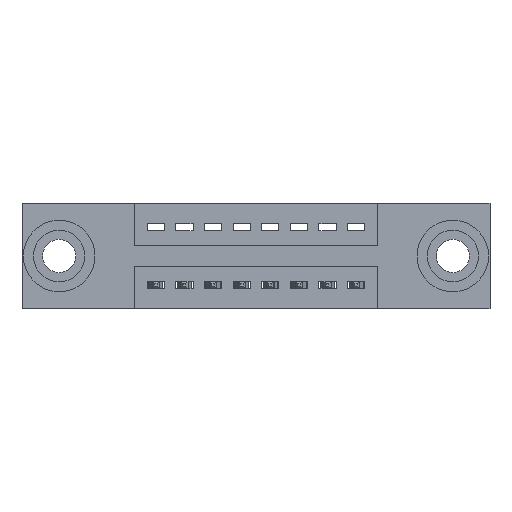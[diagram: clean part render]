
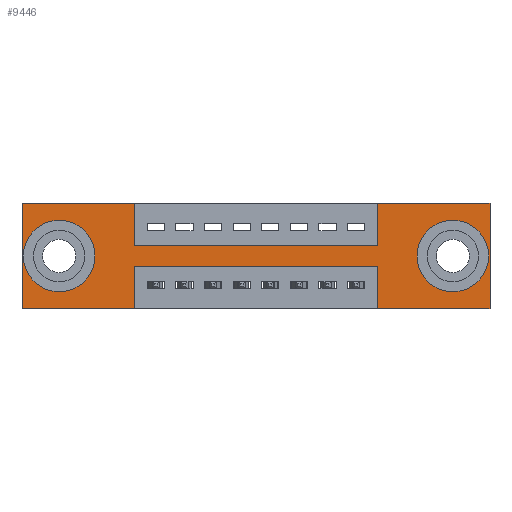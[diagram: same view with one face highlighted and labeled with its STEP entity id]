
A CAD part, front view. The second image highlights one B-rep face of the part: STEP entity #9446.
In plain terms, the highlighted planar face has unit normal (0, -1, 0).
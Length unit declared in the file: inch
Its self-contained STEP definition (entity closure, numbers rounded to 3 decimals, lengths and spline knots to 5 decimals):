
#60 = VERTEX_POINT ( 'NONE', #6578 ) ;
#128 = DIRECTION ( 'NONE',  ( 0., 0., -1. ) ) ;
#153 = VERTEX_POINT ( 'NONE', #2269 ) ;
#289 = CARTESIAN_POINT ( 'NONE',  ( 0.3925, 0., -0.37 ) ) ;
#307 = VERTEX_POINT ( 'NONE', #1659 ) ;
#315 = CARTESIAN_POINT ( 'NONE',  ( 0.3925, 0., -0.15 ) ) ;
#331 = DIRECTION ( 'NONE',  ( 0., 0., 1. ) ) ;
#433 = EDGE_LOOP ( 'NONE', ( #3900, #6845 ) ) ;
#526 = LINE ( 'NONE', #1636, #4480 ) ;
#568 = CARTESIAN_POINT ( 'NONE',  ( 0., 0., 0. ) ) ;
#643 = CARTESIAN_POINT ( 'NONE',  ( 0.3925, 0., 0. ) ) ;
#735 = ORIENTED_EDGE ( 'NONE', *, *, #931, .T. ) ;
#931 = EDGE_CURVE ( 'NONE', #4063, #60, #10471, .T. ) ;
#942 = ORIENTED_EDGE ( 'NONE', *, *, #6982, .F. ) ;
#1045 = ORIENTED_EDGE ( 'NONE', *, *, #2650, .F. ) ;
#1110 = DIRECTION ( 'NONE',  ( 0., 0., -1. ) ) ;
#1245 = CARTESIAN_POINT ( 'NONE',  ( 1.635, 0., -0.37 ) ) ;
#1304 = VERTEX_POINT ( 'NONE', #8919 ) ;
#1343 = CARTESIAN_POINT ( 'NONE',  ( 1.2425, 0., 0. ) ) ;
#1618 = CARTESIAN_POINT ( 'NONE',  ( 0.3925, 0., -0.22 ) ) ;
#1636 = CARTESIAN_POINT ( 'NONE',  ( 0., 0., 0. ) ) ;
#1659 = CARTESIAN_POINT ( 'NONE',  ( 1.2425, 0., -0.37 ) ) ;
#1731 = DIRECTION ( 'NONE',  ( -1., 0., 0. ) ) ;
#1753 = VECTOR ( 'NONE', #4052, 39.37008 ) ;
#1759 = ORIENTED_EDGE ( 'NONE', *, *, #3820, .F. ) ;
#1963 = DIRECTION ( 'NONE',  ( 1., 0., 0. ) ) ;
#1981 = CARTESIAN_POINT ( 'NONE',  ( 1.505, 0., -0.185 ) ) ;
#2000 = CARTESIAN_POINT ( 'NONE',  ( 0.13, 0., -0.107 ) ) ;
#2029 = DIRECTION ( 'NONE',  ( -1., 0., 0. ) ) ;
#2114 = LINE ( 'NONE', #1618, #9882 ) ;
#2201 = ORIENTED_EDGE ( 'NONE', *, *, #4584, .F. ) ;
#2204 = DIRECTION ( 'NONE',  ( 0., 0., 1. ) ) ;
#2269 = CARTESIAN_POINT ( 'NONE',  ( 1.2425, 0., -0.15 ) ) ;
#2284 = FACE_BOUND ( 'NONE', #433, .T. ) ;
#2317 = LINE ( 'NONE', #9646, #4358 ) ;
#2338 = DIRECTION ( 'NONE',  ( 0., 0., -1. ) ) ;
#2351 = VECTOR ( 'NONE', #2029, 39.37008 ) ;
#2459 = DIRECTION ( 'NONE',  ( 1., 0., 0. ) ) ;
#2521 = EDGE_LOOP ( 'NONE', ( #5849, #1045, #10937, #2791, #942, #10376, #9166, #8286, #11074, #4075, #2201, #1759 ) ) ;
#2650 = EDGE_CURVE ( 'NONE', #6185, #4301, #2114, .T. ) ;
#2688 = DIRECTION ( 'NONE',  ( 0., 0., 1. ) ) ;
#2727 = CARTESIAN_POINT ( 'NONE',  ( 0.13, 0., -0.185 ) ) ;
#2745 = LINE ( 'NONE', #315, #7666 ) ;
#2784 = CARTESIAN_POINT ( 'NONE',  ( 1.2425, 0., -0.37 ) ) ;
#2791 = ORIENTED_EDGE ( 'NONE', *, *, #5327, .F. ) ;
#3038 = VERTEX_POINT ( 'NONE', #1245 ) ;
#3396 = VECTOR ( 'NONE', #2204, 39.37008 ) ;
#3820 = EDGE_CURVE ( 'NONE', #10307, #1304, #5655, .T. ) ;
#3857 = EDGE_CURVE ( 'NONE', #6645, #8195, #11081, .T. ) ;
#3900 = ORIENTED_EDGE ( 'NONE', *, *, #8445, .T. ) ;
#3925 = LINE ( 'NONE', #2784, #8863 ) ;
#4052 = DIRECTION ( 'NONE',  ( -1., 0., 0. ) ) ;
#4058 = CARTESIAN_POINT ( 'NONE',  ( 1.505, 0., -0.107 ) ) ;
#4063 = VERTEX_POINT ( 'NONE', #2000 ) ;
#4065 = LINE ( 'NONE', #8425, #1753 ) ;
#4075 = ORIENTED_EDGE ( 'NONE', *, *, #8990, .F. ) ;
#4301 = VERTEX_POINT ( 'NONE', #6123 ) ;
#4358 = VECTOR ( 'NONE', #11283, 39.37008 ) ;
#4439 = CARTESIAN_POINT ( 'NONE',  ( 0.3925, 0., -0.37 ) ) ;
#4464 = AXIS2_PLACEMENT_3D ( 'NONE', #5809, #7580, #2338 ) ;
#4480 = VECTOR ( 'NONE', #2459, 39.37008 ) ;
#4584 = EDGE_CURVE ( 'NONE', #1304, #7609, #8911, .T. ) ;
#4637 = EDGE_LOOP ( 'NONE', ( #735, #5672 ) ) ;
#4876 = AXIS2_PLACEMENT_3D ( 'NONE', #10979, #5778, #6798 ) ;
#4888 = PLANE ( 'NONE',  #4876 ) ;
#5173 = AXIS2_PLACEMENT_3D ( 'NONE', #1981, #10635, #128 ) ;
#5235 = VERTEX_POINT ( 'NONE', #643 ) ;
#5327 = EDGE_CURVE ( 'NONE', #3038, #307, #4065, .T. ) ;
#5449 = DIRECTION ( 'NONE',  ( 0., 0., 1. ) ) ;
#5454 = DIRECTION ( 'NONE',  ( 1., 0., 0. ) ) ;
#5500 = LINE ( 'NONE', #8030, #8903 ) ;
#5539 = DIRECTION ( 'NONE',  ( 0., 1., 0. ) ) ;
#5655 = LINE ( 'NONE', #7265, #2351 ) ;
#5672 = ORIENTED_EDGE ( 'NONE', *, *, #10271, .T. ) ;
#5778 = DIRECTION ( 'NONE',  ( 0., -1., 0. ) ) ;
#5809 = CARTESIAN_POINT ( 'NONE',  ( 1.505, 0., -0.185 ) ) ;
#5849 = ORIENTED_EDGE ( 'NONE', *, *, #6382, .F. ) ;
#5914 = LINE ( 'NONE', #4439, #7551 ) ;
#5947 = VERTEX_POINT ( 'NONE', #9475 ) ;
#6069 = CARTESIAN_POINT ( 'NONE',  ( 0., 0., 0. ) ) ;
#6123 = CARTESIAN_POINT ( 'NONE',  ( 0.3925, 0., -0.22 ) ) ;
#6124 = FACE_BOUND ( 'NONE', #4637, .T. ) ;
#6185 = VERTEX_POINT ( 'NONE', #9201 ) ;
#6382 = EDGE_CURVE ( 'NONE', #4301, #10307, #5914, .T. ) ;
#6578 = CARTESIAN_POINT ( 'NONE',  ( 0.13, 0., -0.263 ) ) ;
#6592 = DIRECTION ( 'NONE',  ( 0., 0., 1. ) ) ;
#6645 = VERTEX_POINT ( 'NONE', #10576 ) ;
#6713 = AXIS2_PLACEMENT_3D ( 'NONE', #2727, #7932, #2688 ) ;
#6780 = VERTEX_POINT ( 'NONE', #9771 ) ;
#6798 = DIRECTION ( 'NONE',  ( 0., 0., -1. ) ) ;
#6845 = ORIENTED_EDGE ( 'NONE', *, *, #3857, .T. ) ;
#6869 = EDGE_CURVE ( 'NONE', #5235, #5947, #2317, .T. ) ;
#6970 = EDGE_CURVE ( 'NONE', #5947, #153, #2745, .T. ) ;
#6982 = EDGE_CURVE ( 'NONE', #6780, #3038, #5500, .T. ) ;
#7009 = AXIS2_PLACEMENT_3D ( 'NONE', #7207, #5539, #331 ) ;
#7207 = CARTESIAN_POINT ( 'NONE',  ( 0.13, 0., -0.185 ) ) ;
#7265 = CARTESIAN_POINT ( 'NONE',  ( 0., 0., -0.37 ) ) ;
#7551 = VECTOR ( 'NONE', #1110, 39.37008 ) ;
#7580 = DIRECTION ( 'NONE',  ( 0., 1., 0. ) ) ;
#7609 = VERTEX_POINT ( 'NONE', #6069 ) ;
#7666 = VECTOR ( 'NONE', #5454, 39.37008 ) ;
#7750 = VECTOR ( 'NONE', #1963, 39.37008 ) ;
#7793 = EDGE_CURVE ( 'NONE', #153, #11178, #10351, .T. ) ;
#7932 = DIRECTION ( 'NONE',  ( 0., 1., 0. ) ) ;
#8030 = CARTESIAN_POINT ( 'NONE',  ( 1.635, 0., 0. ) ) ;
#8040 = LINE ( 'NONE', #9778, #7750 ) ;
#8195 = VERTEX_POINT ( 'NONE', #4058 ) ;
#8241 = EDGE_CURVE ( 'NONE', #11178, #6780, #526, .T. ) ;
#8286 = ORIENTED_EDGE ( 'NONE', *, *, #6970, .F. ) ;
#8425 = CARTESIAN_POINT ( 'NONE',  ( 0., 0., -0.37 ) ) ;
#8445 = EDGE_CURVE ( 'NONE', #8195, #6645, #9944, .T. ) ;
#8529 = EDGE_CURVE ( 'NONE', #307, #6185, #3925, .T. ) ;
#8863 = VECTOR ( 'NONE', #5449, 39.37008 ) ;
#8903 = VECTOR ( 'NONE', #9799, 39.37008 ) ;
#8911 = LINE ( 'NONE', #568, #9838 ) ;
#8919 = CARTESIAN_POINT ( 'NONE',  ( 0., 0., -0.37 ) ) ;
#8990 = EDGE_CURVE ( 'NONE', #7609, #5235, #8040, .T. ) ;
#9122 = FACE_OUTER_BOUND ( 'NONE', #2521, .T. ) ;
#9166 = ORIENTED_EDGE ( 'NONE', *, *, #7793, .F. ) ;
#9201 = CARTESIAN_POINT ( 'NONE',  ( 1.2425, 0., -0.22 ) ) ;
#9446 = ADVANCED_FACE ( 'NONE', ( #2284, #6124, #9122 ), #4888, .T. ) ;
#9475 = CARTESIAN_POINT ( 'NONE',  ( 0.3925, 0., -0.15 ) ) ;
#9646 = CARTESIAN_POINT ( 'NONE',  ( 0.3925, 0., 0. ) ) ;
#9771 = CARTESIAN_POINT ( 'NONE',  ( 1.635, 0., 0. ) ) ;
#9778 = CARTESIAN_POINT ( 'NONE',  ( 0., 0., 0. ) ) ;
#9799 = DIRECTION ( 'NONE',  ( 0., 0., -1. ) ) ;
#9838 = VECTOR ( 'NONE', #6592, 39.37008 ) ;
#9882 = VECTOR ( 'NONE', #1731, 39.37008 ) ;
#9944 = CIRCLE ( 'NONE', #5173, 0.078 ) ;
#10029 = CIRCLE ( 'NONE', #7009, 0.078 ) ;
#10271 = EDGE_CURVE ( 'NONE', #60, #4063, #10029, .T. ) ;
#10307 = VERTEX_POINT ( 'NONE', #289 ) ;
#10351 = LINE ( 'NONE', #1343, #3396 ) ;
#10376 = ORIENTED_EDGE ( 'NONE', *, *, #8241, .F. ) ;
#10471 = CIRCLE ( 'NONE', #6713, 0.078 ) ;
#10576 = CARTESIAN_POINT ( 'NONE',  ( 1.505, 0., -0.263 ) ) ;
#10635 = DIRECTION ( 'NONE',  ( 0., 1., 0. ) ) ;
#10836 = CARTESIAN_POINT ( 'NONE',  ( 1.2425, 0., 0. ) ) ;
#10937 = ORIENTED_EDGE ( 'NONE', *, *, #8529, .F. ) ;
#10979 = CARTESIAN_POINT ( 'NONE',  ( 0., 0., -0.37 ) ) ;
#11074 = ORIENTED_EDGE ( 'NONE', *, *, #6869, .F. ) ;
#11081 = CIRCLE ( 'NONE', #4464, 0.078 ) ;
#11178 = VERTEX_POINT ( 'NONE', #10836 ) ;
#11283 = DIRECTION ( 'NONE',  ( 0., 0., -1. ) ) ;
